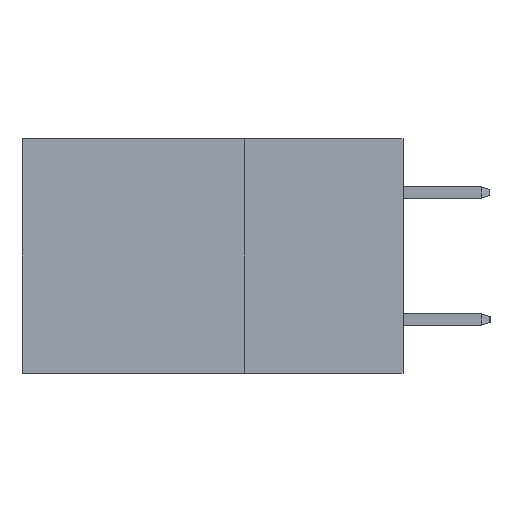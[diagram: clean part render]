
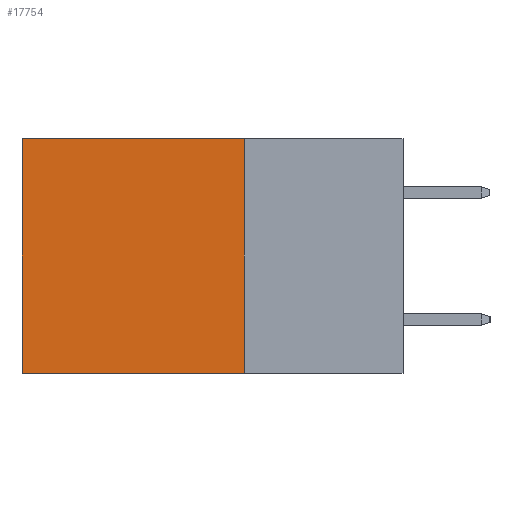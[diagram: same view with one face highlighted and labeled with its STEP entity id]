
A CAD part, left-side view. The second image highlights one B-rep face of the part: STEP entity #17754.
In plain terms, the highlighted planar face has unit normal (-1, 0, 0).
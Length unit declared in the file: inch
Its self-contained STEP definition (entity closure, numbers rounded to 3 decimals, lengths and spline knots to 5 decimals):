
#515 = CARTESIAN_POINT ( 'NONE',  ( 0.2875, 0.25, -0.37 ) ) ;
#1310 = LINE ( 'NONE', #14012, #7855 ) ;
#2357 = VERTEX_POINT ( 'NONE', #10743 ) ;
#3535 = DIRECTION ( 'NONE',  ( 0., 1., 0. ) ) ;
#4094 = ORIENTED_EDGE ( 'NONE', *, *, #5132, .F. ) ;
#4987 = DIRECTION ( 'NONE',  ( 0., 0., -1. ) ) ;
#5132 = EDGE_CURVE ( 'NONE', #17090, #2357, #9539, .T. ) ;
#5283 = CARTESIAN_POINT ( 'NONE',  ( 0.2875, 0.25, 0. ) ) ;
#5398 = LINE ( 'NONE', #15630, #14677 ) ;
#5461 = CARTESIAN_POINT ( 'NONE',  ( 0.2875, 0.6, -0.37 ) ) ;
#6683 = VECTOR ( 'NONE', #11410, 39.37008 ) ;
#7002 = DIRECTION ( 'NONE',  ( 0., 1., 0. ) ) ;
#7007 = DIRECTION ( 'NONE',  ( 0., 0., -1. ) ) ;
#7612 = EDGE_LOOP ( 'NONE', ( #9516, #10081, #4094, #11113 ) ) ;
#7855 = VECTOR ( 'NONE', #7002, 39.37008 ) ;
#8638 = VERTEX_POINT ( 'NONE', #13593 ) ;
#9055 = PLANE ( 'NONE',  #13892 ) ;
#9516 = ORIENTED_EDGE ( 'NONE', *, *, #15624, .T. ) ;
#9539 = LINE ( 'NONE', #5283, #6683 ) ;
#9979 = EDGE_CURVE ( 'NONE', #2357, #14435, #15108, .T. ) ;
#10081 = ORIENTED_EDGE ( 'NONE', *, *, #9979, .F. ) ;
#10743 = CARTESIAN_POINT ( 'NONE',  ( 0.2875, 0.25, -0.37 ) ) ;
#10843 = CARTESIAN_POINT ( 'NONE',  ( 0.2875, 0.25, 0. ) ) ;
#11113 = ORIENTED_EDGE ( 'NONE', *, *, #14006, .T. ) ;
#11410 = DIRECTION ( 'NONE',  ( 0., 0., -1. ) ) ;
#13593 = CARTESIAN_POINT ( 'NONE',  ( 0.2875, 0.6, 0. ) ) ;
#13892 = AXIS2_PLACEMENT_3D ( 'NONE', #10843, #15032, #4987 ) ;
#14006 = EDGE_CURVE ( 'NONE', #17090, #8638, #1310, .T. ) ;
#14012 = CARTESIAN_POINT ( 'NONE',  ( 0.2875, 0.25, 0. ) ) ;
#14435 = VERTEX_POINT ( 'NONE', #5461 ) ;
#14582 = CARTESIAN_POINT ( 'NONE',  ( 0.2875, 0.25, 0. ) ) ;
#14677 = VECTOR ( 'NONE', #7007, 39.37008 ) ;
#15000 = VECTOR ( 'NONE', #3535, 39.37008 ) ;
#15032 = DIRECTION ( 'NONE',  ( 1., 0., 0. ) ) ;
#15108 = LINE ( 'NONE', #515, #15000 ) ;
#15624 = EDGE_CURVE ( 'NONE', #8638, #14435, #5398, .T. ) ;
#15630 = CARTESIAN_POINT ( 'NONE',  ( 0.2875, 0.6, 0. ) ) ;
#16462 = FACE_OUTER_BOUND ( 'NONE', #7612, .T. ) ;
#17090 = VERTEX_POINT ( 'NONE', #14582 ) ;
#17754 = ADVANCED_FACE ( 'NONE', ( #16462 ), #9055, .F. ) ;
